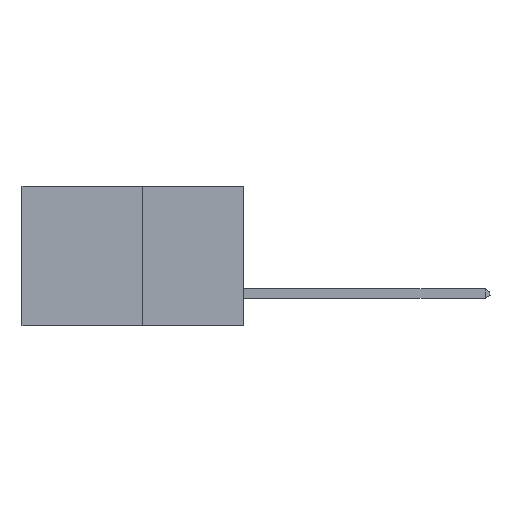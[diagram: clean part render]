
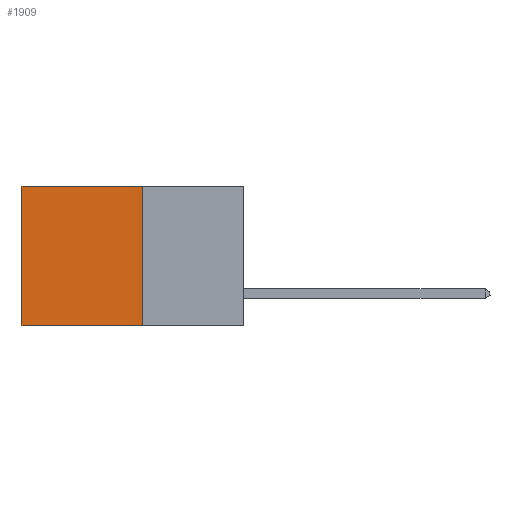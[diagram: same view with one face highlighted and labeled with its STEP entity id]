
A CAD part, left-side view. The second image highlights one B-rep face of the part: STEP entity #1909.
In plain terms, the highlighted planar face has unit normal (-1, 0, 0).
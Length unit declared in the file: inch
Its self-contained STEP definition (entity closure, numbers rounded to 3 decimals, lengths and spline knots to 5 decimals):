
#364 = CARTESIAN_POINT ( 'NONE',  ( 0.277, 0.59, -0.37 ) ) ;
#406 = VECTOR ( 'NONE', #6022, 39.37008 ) ;
#1234 = EDGE_CURVE ( 'NONE', #4449, #5122, #2372, .T. ) ;
#1890 = ORIENTED_EDGE ( 'NONE', *, *, #4946, .T. ) ;
#1909 = ADVANCED_FACE ( 'NONE', ( #2259 ), #6235, .F. ) ;
#1993 = ORIENTED_EDGE ( 'NONE', *, *, #4396, .F. ) ;
#2072 = AXIS2_PLACEMENT_3D ( 'NONE', #5787, #2492, #7347 ) ;
#2155 = VECTOR ( 'NONE', #7480, 39.37008 ) ;
#2259 = FACE_OUTER_BOUND ( 'NONE', #2659, .T. ) ;
#2316 = LINE ( 'NONE', #5612, #406 ) ;
#2372 = LINE ( 'NONE', #7555, #2155 ) ;
#2465 = ORIENTED_EDGE ( 'NONE', *, *, #6289, .T. ) ;
#2492 = DIRECTION ( 'NONE',  ( 1., 0., 0. ) ) ;
#2659 = EDGE_LOOP ( 'NONE', ( #1890, #1993, #7387, #2465 ) ) ;
#3077 = CARTESIAN_POINT ( 'NONE',  ( 0.277, 0.27, 0. ) ) ;
#3360 = DIRECTION ( 'NONE',  ( 0., 1., 0. ) ) ;
#3762 = CARTESIAN_POINT ( 'NONE',  ( 0.277, 0.27, -0.37 ) ) ;
#4296 = LINE ( 'NONE', #6309, #7950 ) ;
#4396 = EDGE_CURVE ( 'NONE', #5122, #5182, #5594, .T. ) ;
#4449 = VERTEX_POINT ( 'NONE', #3077 ) ;
#4946 = EDGE_CURVE ( 'NONE', #5997, #5182, #4296, .T. ) ;
#5122 = VERTEX_POINT ( 'NONE', #6288 ) ;
#5182 = VERTEX_POINT ( 'NONE', #364 ) ;
#5594 = LINE ( 'NONE', #3762, #8997 ) ;
#5612 = CARTESIAN_POINT ( 'NONE',  ( 0.277, 0.27, 0. ) ) ;
#5787 = CARTESIAN_POINT ( 'NONE',  ( 0.277, 0.27, -0.37 ) ) ;
#5997 = VERTEX_POINT ( 'NONE', #7176 ) ;
#6022 = DIRECTION ( 'NONE',  ( 0., 1., 0. ) ) ;
#6235 = PLANE ( 'NONE',  #2072 ) ;
#6288 = CARTESIAN_POINT ( 'NONE',  ( 0.277, 0.27, -0.37 ) ) ;
#6289 = EDGE_CURVE ( 'NONE', #4449, #5997, #2316, .T. ) ;
#6309 = CARTESIAN_POINT ( 'NONE',  ( 0.277, 0.59, -0.37 ) ) ;
#6964 = DIRECTION ( 'NONE',  ( 0., 0., -1. ) ) ;
#7176 = CARTESIAN_POINT ( 'NONE',  ( 0.277, 0.59, 0. ) ) ;
#7347 = DIRECTION ( 'NONE',  ( 0., 0., -1. ) ) ;
#7387 = ORIENTED_EDGE ( 'NONE', *, *, #1234, .F. ) ;
#7480 = DIRECTION ( 'NONE',  ( 0., 0., -1. ) ) ;
#7555 = CARTESIAN_POINT ( 'NONE',  ( 0.277, 0.27, -0.37 ) ) ;
#7950 = VECTOR ( 'NONE', #6964, 39.37008 ) ;
#8997 = VECTOR ( 'NONE', #3360, 39.37008 ) ;
